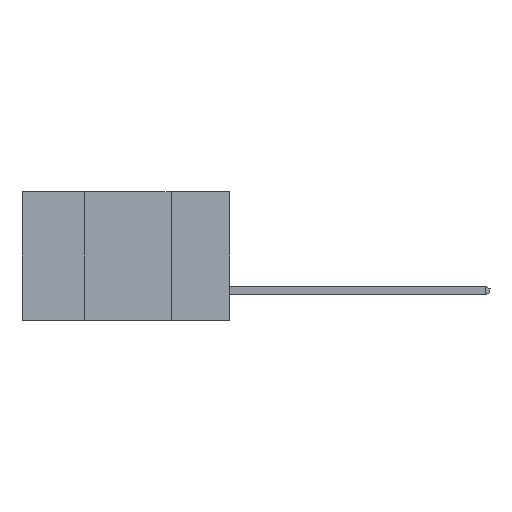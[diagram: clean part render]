
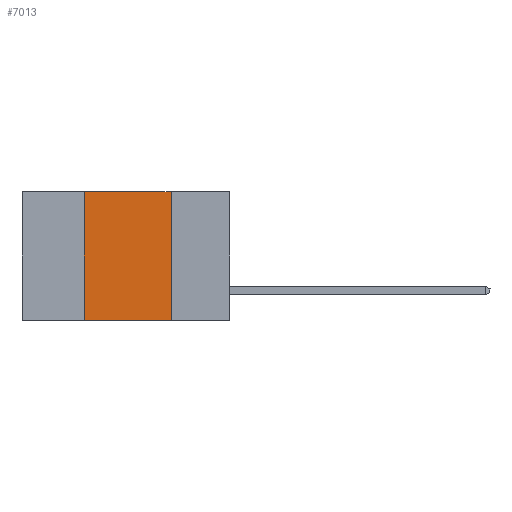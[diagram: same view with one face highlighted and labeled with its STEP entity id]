
A CAD part, left-side view. The second image highlights one B-rep face of the part: STEP entity #7013.
In plain terms, the highlighted planar face has unit normal (-1, 0, 0).
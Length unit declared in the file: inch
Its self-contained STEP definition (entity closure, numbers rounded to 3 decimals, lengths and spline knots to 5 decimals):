
#713 = VECTOR ( 'NONE', #5672, 39.37008 ) ;
#777 = LINE ( 'NONE', #4113, #9463 ) ;
#1325 = EDGE_CURVE ( 'NONE', #7643, #8385, #2382, .T. ) ;
#1341 = EDGE_CURVE ( 'NONE', #3290, #7643, #777, .T. ) ;
#1554 = ORIENTED_EDGE ( 'NONE', *, *, #1325, .F. ) ;
#2142 = EDGE_CURVE ( 'NONE', #8385, #5372, #7694, .T. ) ;
#2241 = ORIENTED_EDGE ( 'NONE', *, *, #2142, .F. ) ;
#2276 = CARTESIAN_POINT ( 'NONE',  ( 0., 0.6, 0. ) ) ;
#2382 = LINE ( 'NONE', #4063, #713 ) ;
#2530 = VECTOR ( 'NONE', #5611, 39.37008 ) ;
#3165 = EDGE_CURVE ( 'NONE', #3290, #5372, #4807, .T. ) ;
#3290 = VERTEX_POINT ( 'NONE', #8133 ) ;
#3520 = CARTESIAN_POINT ( 'NONE',  ( 0., 0.17, 0. ) ) ;
#4063 = CARTESIAN_POINT ( 'NONE',  ( 0., 0.6, 0. ) ) ;
#4113 = CARTESIAN_POINT ( 'NONE',  ( 0., 0.42, -0.37 ) ) ;
#4807 = LINE ( 'NONE', #7865, #2530 ) ;
#4927 = DIRECTION ( 'NONE',  ( 0., 0., 1. ) ) ;
#5372 = VERTEX_POINT ( 'NONE', #8857 ) ;
#5511 = FACE_OUTER_BOUND ( 'NONE', #8493, .T. ) ;
#5611 = DIRECTION ( 'NONE',  ( 0., -1., 0. ) ) ;
#5672 = DIRECTION ( 'NONE',  ( 0., -1., 0. ) ) ;
#5950 = VECTOR ( 'NONE', #10109, 39.37008 ) ;
#6129 = CARTESIAN_POINT ( 'NONE',  ( 0., 0.17, -0.37 ) ) ;
#6523 = AXIS2_PLACEMENT_3D ( 'NONE', #2276, #8024, #7172 ) ;
#7013 = ADVANCED_FACE ( 'NONE', ( #5511 ), #7925, .F. ) ;
#7172 = DIRECTION ( 'NONE',  ( 0., 0., -1. ) ) ;
#7569 = CARTESIAN_POINT ( 'NONE',  ( 0., 0.42, 0. ) ) ;
#7643 = VERTEX_POINT ( 'NONE', #7569 ) ;
#7694 = LINE ( 'NONE', #6129, #5950 ) ;
#7762 = ORIENTED_EDGE ( 'NONE', *, *, #1341, .F. ) ;
#7865 = CARTESIAN_POINT ( 'NONE',  ( 0., 0.6, -0.37 ) ) ;
#7925 = PLANE ( 'NONE',  #6523 ) ;
#8024 = DIRECTION ( 'NONE',  ( 1., 0., 0. ) ) ;
#8133 = CARTESIAN_POINT ( 'NONE',  ( 0., 0.42, -0.37 ) ) ;
#8385 = VERTEX_POINT ( 'NONE', #3520 ) ;
#8493 = EDGE_LOOP ( 'NONE', ( #2241, #1554, #7762, #8708 ) ) ;
#8708 = ORIENTED_EDGE ( 'NONE', *, *, #3165, .T. ) ;
#8857 = CARTESIAN_POINT ( 'NONE',  ( 0., 0.17, -0.37 ) ) ;
#9463 = VECTOR ( 'NONE', #4927, 39.37008 ) ;
#10109 = DIRECTION ( 'NONE',  ( 0., 0., -1. ) ) ;
